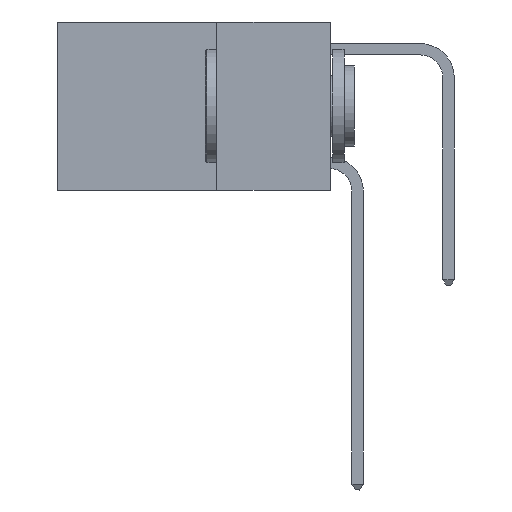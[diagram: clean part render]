
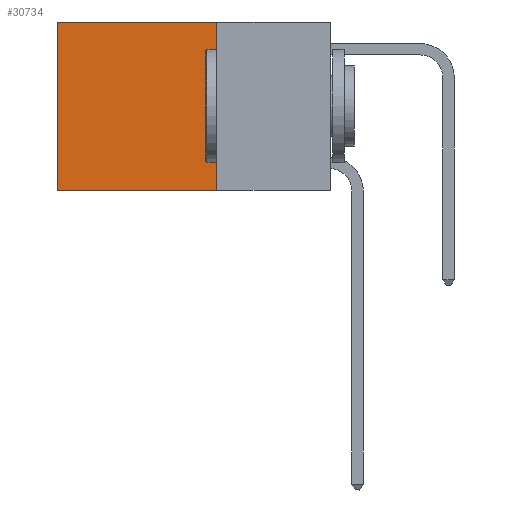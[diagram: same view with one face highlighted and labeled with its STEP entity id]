
A CAD part, left-side view. The second image highlights one B-rep face of the part: STEP entity #30734.
In plain terms, the highlighted planar face has unit normal (-1, 0, 0).
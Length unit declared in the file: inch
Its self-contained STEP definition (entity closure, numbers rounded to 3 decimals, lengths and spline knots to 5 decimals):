
#330 = ORIENTED_EDGE ( 'NONE', *, *, #27029, .F. ) ;
#828 = VERTEX_POINT ( 'NONE', #30405 ) ;
#1608 = CARTESIAN_POINT ( 'NONE',  ( 0.2625, 0.25, 0. ) ) ;
#3686 = PLANE ( 'NONE',  #4693 ) ;
#4026 = DIRECTION ( 'NONE',  ( 1., 0., 0. ) ) ;
#4693 = AXIS2_PLACEMENT_3D ( 'NONE', #8639, #4026, #10927 ) ;
#4850 = CARTESIAN_POINT ( 'NONE',  ( 0.2625, 0.25, 0. ) ) ;
#5554 = CARTESIAN_POINT ( 'NONE',  ( 0.2625, 0.25, -0.37 ) ) ;
#5708 = LINE ( 'NONE', #5554, #19617 ) ;
#5991 = EDGE_CURVE ( 'NONE', #828, #8335, #5708, .T. ) ;
#6705 = DIRECTION ( 'NONE',  ( 0., 1., 0. ) ) ;
#7996 = EDGE_CURVE ( 'NONE', #25474, #8335, #10924, .T. ) ;
#8335 = VERTEX_POINT ( 'NONE', #28464 ) ;
#8639 = CARTESIAN_POINT ( 'NONE',  ( 0.2625, 0.25, 0. ) ) ;
#9857 = ORIENTED_EDGE ( 'NONE', *, *, #32294, .T. ) ;
#10220 = VECTOR ( 'NONE', #21624, 39.37008 ) ;
#10924 = LINE ( 'NONE', #11091, #10220 ) ;
#10927 = DIRECTION ( 'NONE',  ( 0., 0., -1. ) ) ;
#11091 = CARTESIAN_POINT ( 'NONE',  ( 0.2625, 0.6, 0. ) ) ;
#11889 = ORIENTED_EDGE ( 'NONE', *, *, #7996, .T. ) ;
#13195 = CARTESIAN_POINT ( 'NONE',  ( 0.2625, 0.25, 0. ) ) ;
#15860 = VERTEX_POINT ( 'NONE', #13195 ) ;
#17758 = DIRECTION ( 'NONE',  ( 0., 1., 0. ) ) ;
#19617 = VECTOR ( 'NONE', #17758, 39.37008 ) ;
#21190 = VECTOR ( 'NONE', #31471, 39.37008 ) ;
#21624 = DIRECTION ( 'NONE',  ( 0., 0., -1. ) ) ;
#22401 = ORIENTED_EDGE ( 'NONE', *, *, #5991, .F. ) ;
#25266 = VECTOR ( 'NONE', #6705, 39.37008 ) ;
#25474 = VERTEX_POINT ( 'NONE', #28121 ) ;
#26220 = FACE_OUTER_BOUND ( 'NONE', #26823, .T. ) ;
#26823 = EDGE_LOOP ( 'NONE', ( #11889, #22401, #330, #9857 ) ) ;
#27029 = EDGE_CURVE ( 'NONE', #15860, #828, #28876, .T. ) ;
#28121 = CARTESIAN_POINT ( 'NONE',  ( 0.2625, 0.6, 0. ) ) ;
#28464 = CARTESIAN_POINT ( 'NONE',  ( 0.2625, 0.6, -0.37 ) ) ;
#28876 = LINE ( 'NONE', #4850, #21190 ) ;
#30405 = CARTESIAN_POINT ( 'NONE',  ( 0.2625, 0.25, -0.37 ) ) ;
#30734 = ADVANCED_FACE ( 'NONE', ( #26220 ), #3686, .F. ) ;
#31471 = DIRECTION ( 'NONE',  ( 0., 0., -1. ) ) ;
#31956 = LINE ( 'NONE', #1608, #25266 ) ;
#32294 = EDGE_CURVE ( 'NONE', #15860, #25474, #31956, .T. ) ;
